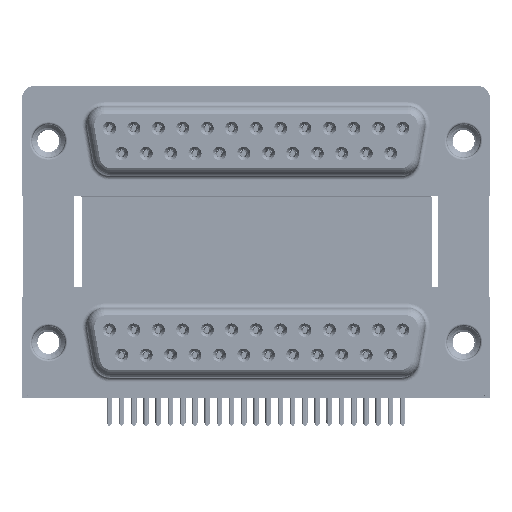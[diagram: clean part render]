
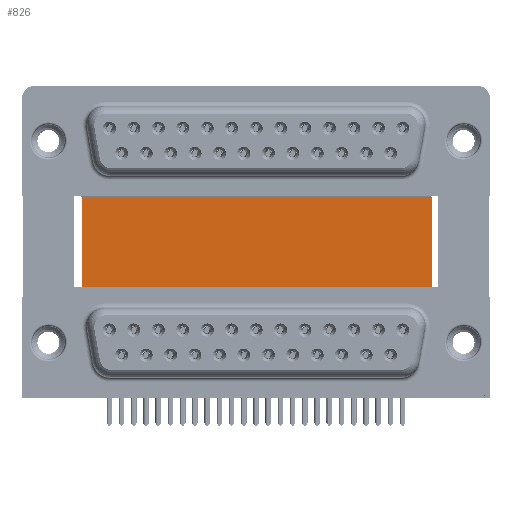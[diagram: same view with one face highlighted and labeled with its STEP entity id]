
A CAD part, top view. The second image highlights one B-rep face of the part: STEP entity #826.
In plain terms, the highlighted planar face has unit normal (0, 0, 1).
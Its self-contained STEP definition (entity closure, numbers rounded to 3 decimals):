
#826 = ADVANCED_FACE ( 'NONE', ( #35752 ), #59641, .F. ) ;
#4422 = EDGE_CURVE ( 'NONE', #7488, #47677, #32463, .T. ) ;
#6442 = CARTESIAN_POINT ( 'NONE',  ( 3.79, 16.585, -12. ) ) ;
#6520 = VECTOR ( 'NONE', #23748, 1000. ) ;
#7488 = VERTEX_POINT ( 'NONE', #23664 ) ;
#8699 = EDGE_CURVE ( 'NONE', #32424, #7488, #31718, .T. ) ;
#17457 = CARTESIAN_POINT ( 'NONE',  ( 43.43, 16.585, -12. ) ) ;
#18020 = CARTESIAN_POINT ( 'NONE',  ( 43.43, -3.735, -12. ) ) ;
#19328 = LINE ( 'NONE', #28582, #62672 ) ;
#21025 = VECTOR ( 'NONE', #51871, 1000. ) ;
#22549 = DIRECTION ( 'NONE',  ( 0., -1., 0. ) ) ;
#23631 = CARTESIAN_POINT ( 'NONE',  ( 43.43, 16.585, -12. ) ) ;
#23664 = CARTESIAN_POINT ( 'NONE',  ( 3.79, -3.735, -12. ) ) ;
#23748 = DIRECTION ( 'NONE',  ( 0., -1., 0. ) ) ;
#25101 = ORIENTED_EDGE ( 'NONE', *, *, #8699, .T. ) ;
#28582 = CARTESIAN_POINT ( 'NONE',  ( 3.79, 16.585, -12. ) ) ;
#30358 = DIRECTION ( 'NONE',  ( 0., 0., -1. ) ) ;
#30950 = ORIENTED_EDGE ( 'NONE', *, *, #4422, .T. ) ;
#31718 = LINE ( 'NONE', #43806, #6520 ) ;
#32424 = VERTEX_POINT ( 'NONE', #51506 ) ;
#32463 = LINE ( 'NONE', #33420, #21025 ) ;
#33420 = CARTESIAN_POINT ( 'NONE',  ( 3.79, -3.735, -12. ) ) ;
#35752 = FACE_OUTER_BOUND ( 'NONE', #54184, .T. ) ;
#36683 = ORIENTED_EDGE ( 'NONE', *, *, #47181, .F. ) ;
#39161 = AXIS2_PLACEMENT_3D ( 'NONE', #6442, #30358, #54556 ) ;
#41570 = EDGE_CURVE ( 'NONE', #32424, #52132, #19328, .T. ) ;
#43806 = CARTESIAN_POINT ( 'NONE',  ( 3.79, 16.585, -12. ) ) ;
#47181 = EDGE_CURVE ( 'NONE', #52132, #47677, #58947, .T. ) ;
#47677 = VERTEX_POINT ( 'NONE', #18020 ) ;
#49246 = DIRECTION ( 'NONE',  ( 1., 0., 0. ) ) ;
#51506 = CARTESIAN_POINT ( 'NONE',  ( 3.79, 16.585, -12. ) ) ;
#51871 = DIRECTION ( 'NONE',  ( 1., 0., 0. ) ) ;
#52132 = VERTEX_POINT ( 'NONE', #23631 ) ;
#54184 = EDGE_LOOP ( 'NONE', ( #30950, #36683, #58960, #25101 ) ) ;
#54556 = DIRECTION ( 'NONE',  ( -1., 0., 0. ) ) ;
#55821 = VECTOR ( 'NONE', #22549, 1000. ) ;
#58947 = LINE ( 'NONE', #17457, #55821 ) ;
#58960 = ORIENTED_EDGE ( 'NONE', *, *, #41570, .F. ) ;
#59641 = PLANE ( 'NONE',  #39161 ) ;
#62672 = VECTOR ( 'NONE', #49246, 1000. ) ;
